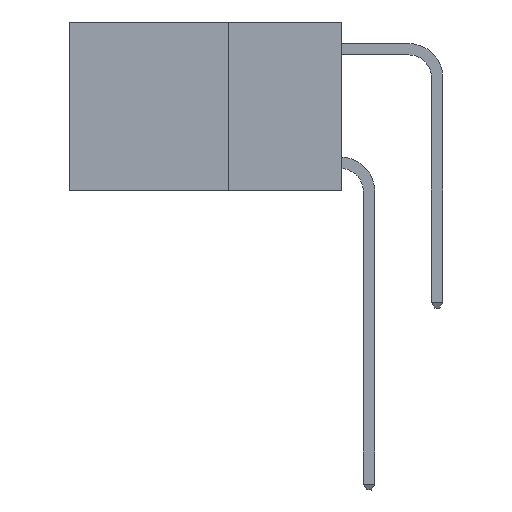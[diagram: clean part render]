
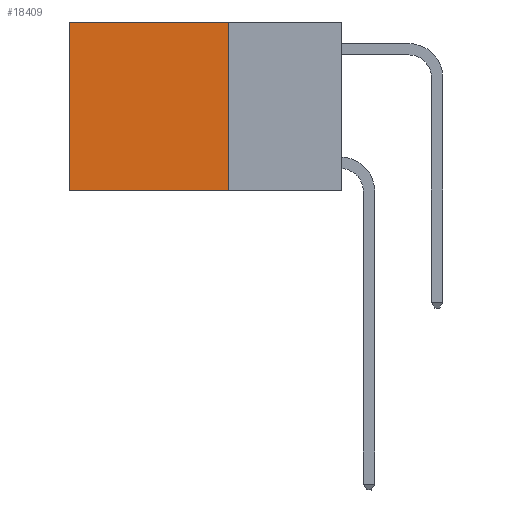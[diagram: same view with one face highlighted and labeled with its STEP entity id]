
A CAD part, left-side view. The second image highlights one B-rep face of the part: STEP entity #18409.
In plain terms, the highlighted planar face has unit normal (-1, 0, 0).
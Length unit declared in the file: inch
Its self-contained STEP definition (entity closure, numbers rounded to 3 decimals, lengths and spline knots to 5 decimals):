
#295 = ORIENTED_EDGE ( 'NONE', *, *, #1185, .F. ) ;
#1185 = EDGE_CURVE ( 'NONE', #15889, #4763, #25749, .T. ) ;
#2785 = DIRECTION ( 'NONE',  ( 0., 1., 0. ) ) ;
#3674 = LINE ( 'NONE', #7356, #15909 ) ;
#4763 = VERTEX_POINT ( 'NONE', #25308 ) ;
#4957 = DIRECTION ( 'NONE',  ( 0., 0., -1. ) ) ;
#5601 = DIRECTION ( 'NONE',  ( 0., 0., -1. ) ) ;
#6945 = FACE_OUTER_BOUND ( 'NONE', #11427, .T. ) ;
#7057 = ORIENTED_EDGE ( 'NONE', *, *, #24299, .T. ) ;
#7356 = CARTESIAN_POINT ( 'NONE',  ( 0.2625, 0.6, 0. ) ) ;
#7463 = VECTOR ( 'NONE', #5601, 39.37008 ) ;
#8033 = VECTOR ( 'NONE', #11914, 39.37008 ) ;
#8508 = CARTESIAN_POINT ( 'NONE',  ( 0.2625, 0.25, -0.37 ) ) ;
#8554 = AXIS2_PLACEMENT_3D ( 'NONE', #24681, #22828, #4957 ) ;
#8869 = VERTEX_POINT ( 'NONE', #13922 ) ;
#9808 = CARTESIAN_POINT ( 'NONE',  ( 0.2625, 0.25, 0. ) ) ;
#10494 = VECTOR ( 'NONE', #2785, 39.37008 ) ;
#10578 = ORIENTED_EDGE ( 'NONE', *, *, #20082, .F. ) ;
#11427 = EDGE_LOOP ( 'NONE', ( #14464, #295, #10578, #7057 ) ) ;
#11914 = DIRECTION ( 'NONE',  ( 0., 1., 0. ) ) ;
#13922 = CARTESIAN_POINT ( 'NONE',  ( 0.2625, 0.25, 0. ) ) ;
#13946 = LINE ( 'NONE', #9808, #7463 ) ;
#14464 = ORIENTED_EDGE ( 'NONE', *, *, #22765, .T. ) ;
#14603 = PLANE ( 'NONE',  #8554 ) ;
#15808 = CARTESIAN_POINT ( 'NONE',  ( 0.2625, 0.25, -0.37 ) ) ;
#15889 = VERTEX_POINT ( 'NONE', #8508 ) ;
#15909 = VECTOR ( 'NONE', #17666, 39.37008 ) ;
#17666 = DIRECTION ( 'NONE',  ( 0., 0., -1. ) ) ;
#18409 = ADVANCED_FACE ( 'NONE', ( #6945 ), #14603, .F. ) ;
#19515 = VERTEX_POINT ( 'NONE', #24845 ) ;
#20082 = EDGE_CURVE ( 'NONE', #8869, #15889, #13946, .T. ) ;
#20662 = CARTESIAN_POINT ( 'NONE',  ( 0.2625, 0.25, 0. ) ) ;
#22765 = EDGE_CURVE ( 'NONE', #19515, #4763, #3674, .T. ) ;
#22828 = DIRECTION ( 'NONE',  ( 1., 0., 0. ) ) ;
#23002 = LINE ( 'NONE', #20662, #10494 ) ;
#24299 = EDGE_CURVE ( 'NONE', #8869, #19515, #23002, .T. ) ;
#24681 = CARTESIAN_POINT ( 'NONE',  ( 0.2625, 0.25, 0. ) ) ;
#24845 = CARTESIAN_POINT ( 'NONE',  ( 0.2625, 0.6, 0. ) ) ;
#25308 = CARTESIAN_POINT ( 'NONE',  ( 0.2625, 0.6, -0.37 ) ) ;
#25749 = LINE ( 'NONE', #15808, #8033 ) ;
